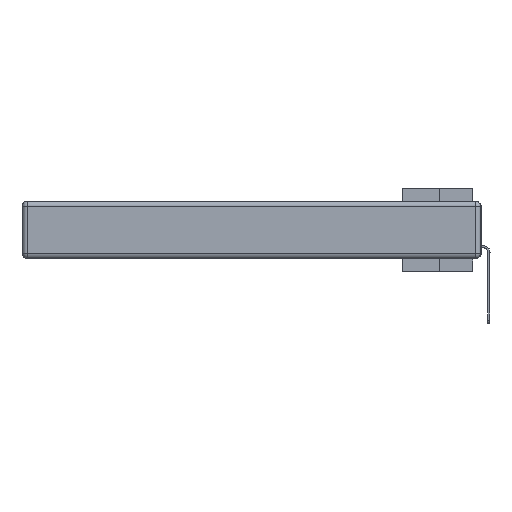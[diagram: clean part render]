
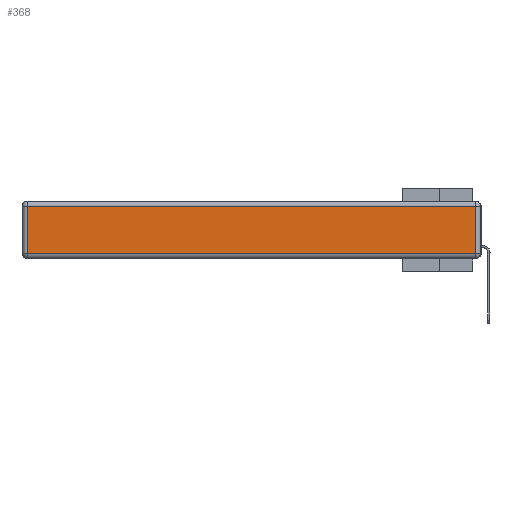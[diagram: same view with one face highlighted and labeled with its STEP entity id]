
A CAD part, left-side view. The second image highlights one B-rep face of the part: STEP entity #368.
In plain terms, the highlighted planar face has unit normal (-1, 0, 0).
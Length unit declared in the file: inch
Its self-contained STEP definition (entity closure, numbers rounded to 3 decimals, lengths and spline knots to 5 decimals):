
#46 = VERTEX_POINT ( 'NONE', #27056 ) ;
#368 = ADVANCED_FACE ( 'NONE', ( #31749 ), #8856, .T. ) ;
#384 = CARTESIAN_POINT ( 'NONE',  ( 0., 2.72, -0.343 ) ) ;
#564 = DIRECTION ( 'NONE',  ( 0., 0., -1. ) ) ;
#1844 = VERTEX_POINT ( 'NONE', #2208 ) ;
#2208 = CARTESIAN_POINT ( 'NONE',  ( 0., 0.03, -0.313 ) ) ;
#2796 = DIRECTION ( 'NONE',  ( -1., 0., 0. ) ) ;
#3221 = LINE ( 'NONE', #384, #31707 ) ;
#3798 = AXIS2_PLACEMENT_3D ( 'NONE', #20205, #2796, #6033 ) ;
#3871 = DIRECTION ( 'NONE',  ( 0., 1., 0. ) ) ;
#5185 = CARTESIAN_POINT ( 'NONE',  ( 0., 0.03, -0.343 ) ) ;
#5684 = ORIENTED_EDGE ( 'NONE', *, *, #11156, .T. ) ;
#6033 = DIRECTION ( 'NONE',  ( 0., 0., 1. ) ) ;
#6364 = LINE ( 'NONE', #29988, #31631 ) ;
#8856 = PLANE ( 'NONE',  #3798 ) ;
#8877 = VERTEX_POINT ( 'NONE', #19874 ) ;
#9764 = EDGE_LOOP ( 'NONE', ( #5684, #20019, #33457, #30003 ) ) ;
#9862 = EDGE_CURVE ( 'NONE', #26556, #8877, #27147, .T. ) ;
#11156 = EDGE_CURVE ( 'NONE', #46, #1844, #6364, .T. ) ;
#15229 = CARTESIAN_POINT ( 'NONE',  ( 0., 2.75, -0.03 ) ) ;
#17274 = LINE ( 'NONE', #5185, #27534 ) ;
#19874 = CARTESIAN_POINT ( 'NONE',  ( 0., 2.72, -0.03 ) ) ;
#20019 = ORIENTED_EDGE ( 'NONE', *, *, #34364, .T. ) ;
#20205 = CARTESIAN_POINT ( 'NONE',  ( 0., 0., -0.343 ) ) ;
#21465 = DIRECTION ( 'NONE',  ( 0., -1., 0. ) ) ;
#26162 = VECTOR ( 'NONE', #3871, 39.37008 ) ;
#26556 = VERTEX_POINT ( 'NONE', #31163 ) ;
#27056 = CARTESIAN_POINT ( 'NONE',  ( 0., 2.72, -0.313 ) ) ;
#27147 = LINE ( 'NONE', #15229, #26162 ) ;
#27534 = VECTOR ( 'NONE', #36623, 39.37008 ) ;
#29988 = CARTESIAN_POINT ( 'NONE',  ( 0., 0., -0.313 ) ) ;
#30003 = ORIENTED_EDGE ( 'NONE', *, *, #33803, .T. ) ;
#31163 = CARTESIAN_POINT ( 'NONE',  ( 0., 0.03, -0.03 ) ) ;
#31631 = VECTOR ( 'NONE', #21465, 39.37008 ) ;
#31707 = VECTOR ( 'NONE', #564, 39.37008 ) ;
#31749 = FACE_OUTER_BOUND ( 'NONE', #9764, .T. ) ;
#33457 = ORIENTED_EDGE ( 'NONE', *, *, #9862, .T. ) ;
#33803 = EDGE_CURVE ( 'NONE', #8877, #46, #3221, .T. ) ;
#34364 = EDGE_CURVE ( 'NONE', #1844, #26556, #17274, .T. ) ;
#36623 = DIRECTION ( 'NONE',  ( 0., 0., 1. ) ) ;
